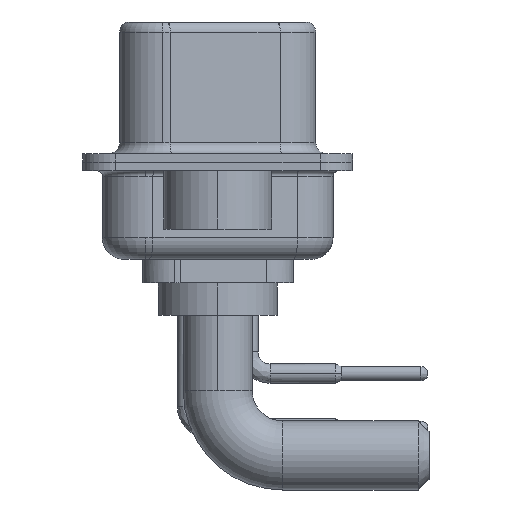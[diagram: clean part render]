
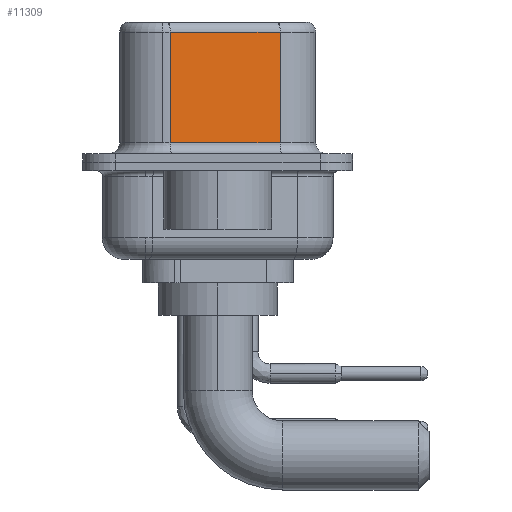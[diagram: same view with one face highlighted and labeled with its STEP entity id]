
A CAD part, left-side view. The second image highlights one B-rep face of the part: STEP entity #11309.
In plain terms, the highlighted planar face has unit normal (-0.985, -0.174, 0).
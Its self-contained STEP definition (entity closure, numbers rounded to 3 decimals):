
#385 = DIRECTION ( 'NONE',  ( 0., 0., -1. ) ) ;
#907 = VECTOR ( 'NONE', #385, 1000. ) ;
#1849 = LINE ( 'NONE', #15856, #14641 ) ;
#3475 = CARTESIAN_POINT ( 'NONE',  ( 3.68, 2.203, 0.9 ) ) ;
#4333 = DIRECTION ( 'NONE',  ( 0., 0., -1. ) ) ;
#4681 = AXIS2_PLACEMENT_3D ( 'NONE', #23197, #22825, #7222 ) ;
#5113 = ORIENTED_EDGE ( 'NONE', *, *, #11927, .T. ) ;
#5764 = DIRECTION ( 'NONE',  ( -0.174, 0.985, 0. ) ) ;
#6285 = CARTESIAN_POINT ( 'NONE',  ( 3.68, 2.203, 6.52 ) ) ;
#6662 = EDGE_CURVE ( 'NONE', #12227, #16573, #9902, .T. ) ;
#6743 = CARTESIAN_POINT ( 'NONE',  ( 4.58, -2.897, 6.52 ) ) ;
#7222 = DIRECTION ( 'NONE',  ( -0.174, 0.985, 0. ) ) ;
#7466 = FACE_OUTER_BOUND ( 'NONE', #19687, .T. ) ;
#7577 = CARTESIAN_POINT ( 'NONE',  ( 4.58, -2.897, 6.02 ) ) ;
#7702 = LINE ( 'NONE', #7577, #18405 ) ;
#9389 = EDGE_CURVE ( 'NONE', #18606, #13422, #12293, .T. ) ;
#9753 = DIRECTION ( 'NONE',  ( 0.174, -0.985, 0. ) ) ;
#9902 = LINE ( 'NONE', #6285, #14101 ) ;
#11309 = ADVANCED_FACE ( 'NONE', ( #7466 ), #11339, .F. ) ;
#11339 = PLANE ( 'NONE',  #4681 ) ;
#11927 = EDGE_CURVE ( 'NONE', #16573, #13422, #1849, .T. ) ;
#12227 = VERTEX_POINT ( 'NONE', #24232 ) ;
#12293 = LINE ( 'NONE', #6743, #907 ) ;
#13422 = VERTEX_POINT ( 'NONE', #22476 ) ;
#14101 = VECTOR ( 'NONE', #4333, 1000. ) ;
#14641 = VECTOR ( 'NONE', #9753, 1000. ) ;
#15856 = CARTESIAN_POINT ( 'NONE',  ( 4.58, -2.897, 0.9 ) ) ;
#16573 = VERTEX_POINT ( 'NONE', #3475 ) ;
#18300 = CARTESIAN_POINT ( 'NONE',  ( 4.58, -2.897, 6.02 ) ) ;
#18405 = VECTOR ( 'NONE', #5764, 1000. ) ;
#18432 = ORIENTED_EDGE ( 'NONE', *, *, #25187, .T. ) ;
#18606 = VERTEX_POINT ( 'NONE', #18300 ) ;
#19687 = EDGE_LOOP ( 'NONE', ( #23667, #18432, #19700, #5113 ) ) ;
#19700 = ORIENTED_EDGE ( 'NONE', *, *, #6662, .T. ) ;
#22476 = CARTESIAN_POINT ( 'NONE',  ( 4.58, -2.897, 0.9 ) ) ;
#22825 = DIRECTION ( 'NONE',  ( 0.985, 0.174, 0. ) ) ;
#23197 = CARTESIAN_POINT ( 'NONE',  ( 4.58, -2.897, 6.52 ) ) ;
#23667 = ORIENTED_EDGE ( 'NONE', *, *, #9389, .F. ) ;
#24232 = CARTESIAN_POINT ( 'NONE',  ( 3.68, 2.203, 6.02 ) ) ;
#25187 = EDGE_CURVE ( 'NONE', #18606, #12227, #7702, .T. ) ;
